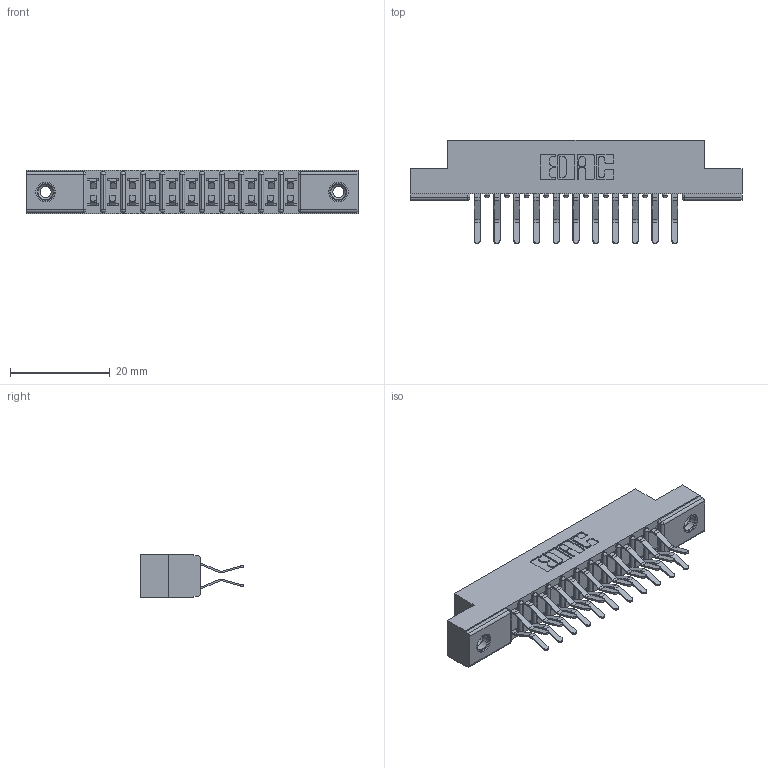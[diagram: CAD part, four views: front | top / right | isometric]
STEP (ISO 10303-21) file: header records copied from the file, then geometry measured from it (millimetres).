
FILE_DESCRIPTION (( 'STEP AP203' ), '1' );
FILE_NAME ('357-022-460-208.STEP', '2020-10-03T00:15:17', ( '' ), ( '' ), 'SwSTEP 2.0', 'SolidWorks 2020', '' );
FILE_SCHEMA (( 'CONFIG_CONTROL_DESIGN' ));
Length unit declared in the file: inch
Products named in the file (4): 307 Part_.156 Dia Mounting Holes; 357-022-460-208; 345-250-001_345-250-003-102; 307-290-001_560
Assembly tree (25 placements, depth 2):
  357-022-460-208
    307 Part_.156 Dia Mounting Holes
    307-290-001_560  x22
    345-250-001_345-250-003-102  x2
Bounding box: 66.6 x 20.73 x 8.71 mm (x, y, z)
Volume: 4378.4 mm3; surface area: 7347.9 mm2
Topology: 25 solids, 25 shells, 1290 faces, 3583 edges, 2318 vertices
Faces by surface type: plane 828, cylinder 422, sphere 24, cone 12, torus 4
Entity records: 14893 total; most frequent: CARTESIAN_POINT 2430, DIRECTION 2403, ORIENTED_EDGE 2398, EDGE_CURVE 1199, LINE 905, VECTOR 905, VERTEX_POINT 776, AXIS2_PLACEMENT_3D 749
